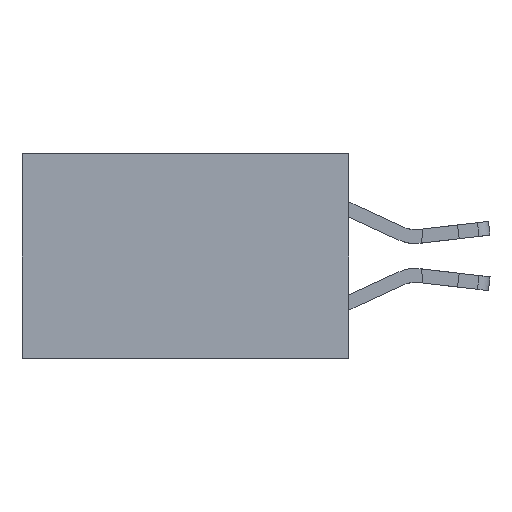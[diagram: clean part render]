
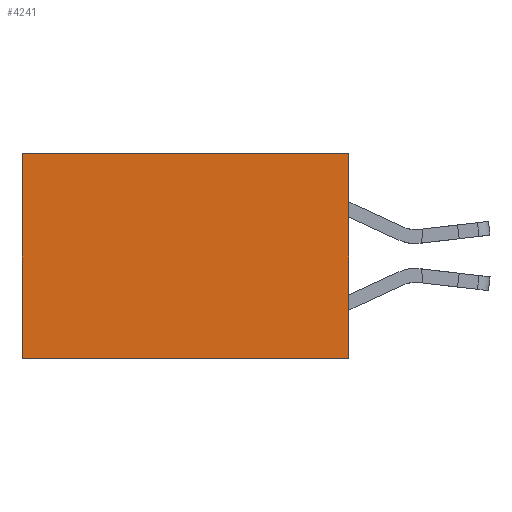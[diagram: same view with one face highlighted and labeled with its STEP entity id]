
A CAD part, left-side view. The second image highlights one B-rep face of the part: STEP entity #4241.
In plain terms, the highlighted planar face has unit normal (-1, 0, 0).
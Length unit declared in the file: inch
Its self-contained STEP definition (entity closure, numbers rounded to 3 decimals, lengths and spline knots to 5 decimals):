
#352 = VERTEX_POINT ( 'NONE', #18977 ) ;
#1215 = EDGE_LOOP ( 'NONE', ( #14423, #22035, #16300, #16843 ) ) ;
#1685 = FACE_OUTER_BOUND ( 'NONE', #1215, .T. ) ;
#1736 = EDGE_CURVE ( 'NONE', #352, #21002, #21530, .T. ) ;
#2986 = VECTOR ( 'NONE', #18724, 39.37008 ) ;
#4241 = ADVANCED_FACE ( 'NONE', ( #1685 ), #20103, .F. ) ;
#4833 = VECTOR ( 'NONE', #19866, 39.37008 ) ;
#8161 = CARTESIAN_POINT ( 'NONE',  ( 0.277, 0., -0.37 ) ) ;
#8970 = CARTESIAN_POINT ( 'NONE',  ( 0.277, 0.59, -0.37 ) ) ;
#10224 = EDGE_CURVE ( 'NONE', #20028, #352, #19874, .T. ) ;
#11152 = VECTOR ( 'NONE', #22819, 39.37008 ) ;
#11383 = AXIS2_PLACEMENT_3D ( 'NONE', #19958, #19899, #19868 ) ;
#11985 = CARTESIAN_POINT ( 'NONE',  ( 0.277, 0., 0. ) ) ;
#13093 = EDGE_CURVE ( 'NONE', #20028, #15249, #22320, .T. ) ;
#14423 = ORIENTED_EDGE ( 'NONE', *, *, #24617, .T. ) ;
#14795 = CARTESIAN_POINT ( 'NONE',  ( 0.277, 0.59, 0. ) ) ;
#15249 = VERTEX_POINT ( 'NONE', #14795 ) ;
#16300 = ORIENTED_EDGE ( 'NONE', *, *, #10224, .F. ) ;
#16843 = ORIENTED_EDGE ( 'NONE', *, *, #13093, .T. ) ;
#17105 = VECTOR ( 'NONE', #24522, 39.37008 ) ;
#18717 = LINE ( 'NONE', #8970, #2986 ) ;
#18724 = DIRECTION ( 'NONE',  ( 0., 0., -1. ) ) ;
#18977 = CARTESIAN_POINT ( 'NONE',  ( 0.277, 0., -0.37 ) ) ;
#19866 = DIRECTION ( 'NONE',  ( 0., 0., -1. ) ) ;
#19868 = DIRECTION ( 'NONE',  ( 0., 0., -1. ) ) ;
#19874 = LINE ( 'NONE', #8161, #4833 ) ;
#19899 = DIRECTION ( 'NONE',  ( 1., 0., 0. ) ) ;
#19958 = CARTESIAN_POINT ( 'NONE',  ( 0.277, 0., -0.37 ) ) ;
#20028 = VERTEX_POINT ( 'NONE', #11985 ) ;
#20103 = PLANE ( 'NONE',  #11383 ) ;
#20995 = CARTESIAN_POINT ( 'NONE',  ( 0.277, 0.59, -0.37 ) ) ;
#21002 = VERTEX_POINT ( 'NONE', #20995 ) ;
#21530 = LINE ( 'NONE', #22576, #11152 ) ;
#22035 = ORIENTED_EDGE ( 'NONE', *, *, #1736, .F. ) ;
#22320 = LINE ( 'NONE', #22634, #17105 ) ;
#22576 = CARTESIAN_POINT ( 'NONE',  ( 0.277, 0., -0.37 ) ) ;
#22634 = CARTESIAN_POINT ( 'NONE',  ( 0.277, 0., 0. ) ) ;
#22819 = DIRECTION ( 'NONE',  ( 0., 1., 0. ) ) ;
#24522 = DIRECTION ( 'NONE',  ( 0., 1., 0. ) ) ;
#24617 = EDGE_CURVE ( 'NONE', #15249, #21002, #18717, .T. ) ;
